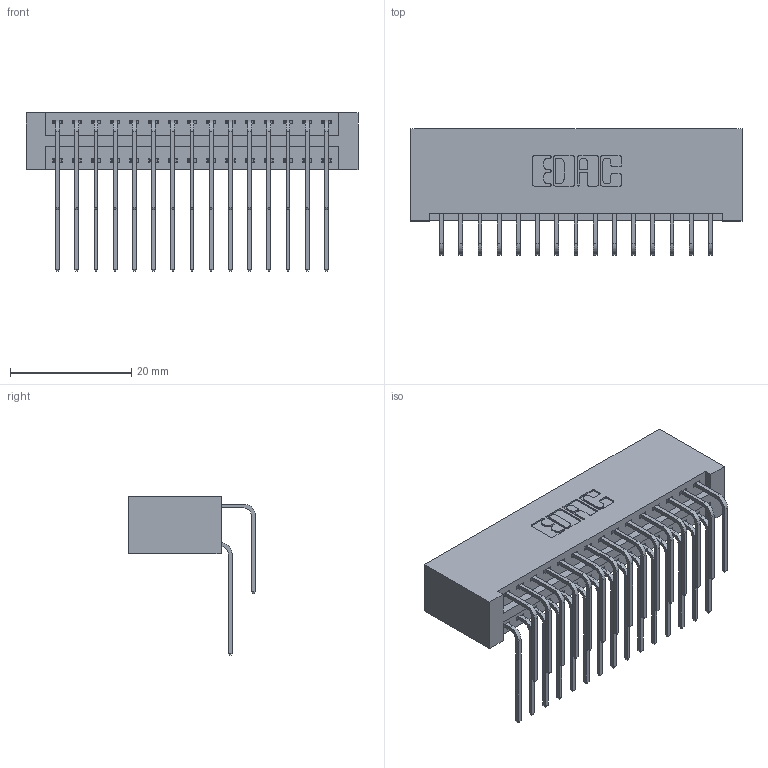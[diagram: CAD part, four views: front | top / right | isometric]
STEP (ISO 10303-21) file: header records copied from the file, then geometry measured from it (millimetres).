
FILE_DESCRIPTION (( 'STEP AP203' ), '1' );
FILE_NAME ('396-030-559-201.STEP', '2018-09-05T08:00:53', ( '' ), ( '' ), 'SwSTEP 2.0', 'SolidWorks 2016', '' );
FILE_SCHEMA (( 'CONFIG_CONTROL_DESIGN' ));
Length unit declared in the file: inch
Products named in the file (4): 346 Part_No Mounting Lugs; 345-292-001_558 559 Tail - 1; 345-292-001_559 Tail - 2; 396-030-559-201
Assembly tree (31 placements, depth 2):
  396-030-559-201
    346 Part_No Mounting Lugs
    345-292-001_558 559 Tail - 1  x15
    345-292-001_559 Tail - 2  x15
Bounding box: 54.86 x 20.89 x 26.16 mm (x, y, z)
Volume: 5886.6 mm3; surface area: 8660.5 mm2
Topology: 31 solids, 31 shells, 1734 faces, 5135 edges, 3382 vertices
Faces by surface type: plane 1182, cylinder 552
Entity records: 14931 total; most frequent: CARTESIAN_POINT 2547, ORIENTED_EDGE 2430, DIRECTION 2263, EDGE_CURVE 1215, LINE 991, VECTOR 991, VERTEX_POINT 806, AXIS2_PLACEMENT_3D 636
